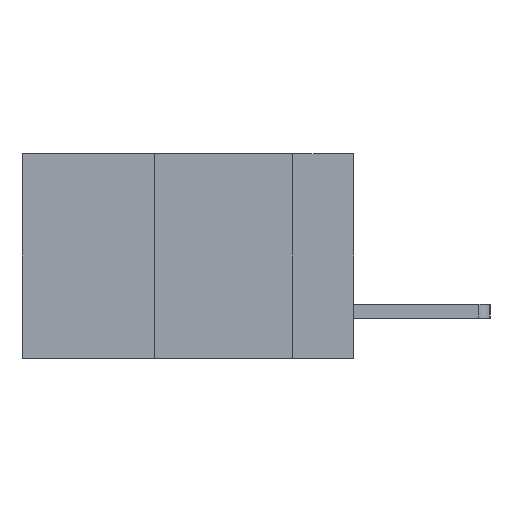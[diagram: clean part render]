
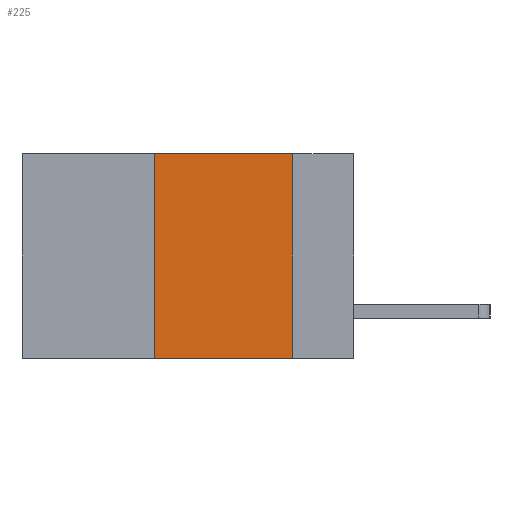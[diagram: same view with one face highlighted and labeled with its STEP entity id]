
A CAD part, left-side view. The second image highlights one B-rep face of the part: STEP entity #225.
In plain terms, the highlighted planar face has unit normal (-1, 0, 0).
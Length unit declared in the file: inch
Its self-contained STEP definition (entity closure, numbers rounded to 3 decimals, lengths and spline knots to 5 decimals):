
#225 = ADVANCED_FACE ( 'NONE', ( #5084 ), #13360, .F. ) ;
#508 = CARTESIAN_POINT ( 'NONE',  ( 0., 0.36, 0. ) ) ;
#1190 = DIRECTION ( 'NONE',  ( 0., -1., 0. ) ) ;
#1969 = VECTOR ( 'NONE', #1190, 39.37008 ) ;
#2049 = CARTESIAN_POINT ( 'NONE',  ( 0., 0.11, -0.37 ) ) ;
#2216 = CARTESIAN_POINT ( 'NONE',  ( 0., 0.6, 0. ) ) ;
#2385 = EDGE_LOOP ( 'NONE', ( #5897, #5555, #12732, #5018 ) ) ;
#2966 = VECTOR ( 'NONE', #7599, 39.37008 ) ;
#3202 = VECTOR ( 'NONE', #5023, 39.37008 ) ;
#4421 = CARTESIAN_POINT ( 'NONE',  ( 0., 0.36, -0.37 ) ) ;
#4956 = VERTEX_POINT ( 'NONE', #9602 ) ;
#5018 = ORIENTED_EDGE ( 'NONE', *, *, #7126, .T. ) ;
#5023 = DIRECTION ( 'NONE',  ( 0., 0., 1. ) ) ;
#5084 = FACE_OUTER_BOUND ( 'NONE', #2385, .T. ) ;
#5555 = ORIENTED_EDGE ( 'NONE', *, *, #13289, .F. ) ;
#5897 = ORIENTED_EDGE ( 'NONE', *, *, #8376, .F. ) ;
#6904 = VECTOR ( 'NONE', #13019, 39.37008 ) ;
#7005 = LINE ( 'NONE', #9621, #3202 ) ;
#7126 = EDGE_CURVE ( 'NONE', #14648, #10246, #10507, .T. ) ;
#7372 = DIRECTION ( 'NONE',  ( 1., 0., 0. ) ) ;
#7599 = DIRECTION ( 'NONE',  ( 0., 0., -1. ) ) ;
#7608 = CARTESIAN_POINT ( 'NONE',  ( 0., 0.6, 0. ) ) ;
#8263 = VERTEX_POINT ( 'NONE', #508 ) ;
#8376 = EDGE_CURVE ( 'NONE', #4956, #10246, #14677, .T. ) ;
#9602 = CARTESIAN_POINT ( 'NONE',  ( 0., 0.11, 0. ) ) ;
#9621 = CARTESIAN_POINT ( 'NONE',  ( 0., 0.36, 0. ) ) ;
#10216 = AXIS2_PLACEMENT_3D ( 'NONE', #7608, #7372, #12174 ) ;
#10246 = VERTEX_POINT ( 'NONE', #2049 ) ;
#10504 = LINE ( 'NONE', #2216, #1969 ) ;
#10507 = LINE ( 'NONE', #12772, #6904 ) ;
#10870 = EDGE_CURVE ( 'NONE', #14648, #8263, #7005, .T. ) ;
#12174 = DIRECTION ( 'NONE',  ( 0., 0., -1. ) ) ;
#12321 = CARTESIAN_POINT ( 'NONE',  ( 0., 0.11, 0. ) ) ;
#12732 = ORIENTED_EDGE ( 'NONE', *, *, #10870, .F. ) ;
#12772 = CARTESIAN_POINT ( 'NONE',  ( 0., 0.6, -0.37 ) ) ;
#13019 = DIRECTION ( 'NONE',  ( 0., -1., 0. ) ) ;
#13289 = EDGE_CURVE ( 'NONE', #8263, #4956, #10504, .T. ) ;
#13360 = PLANE ( 'NONE',  #10216 ) ;
#14648 = VERTEX_POINT ( 'NONE', #4421 ) ;
#14677 = LINE ( 'NONE', #12321, #2966 ) ;
